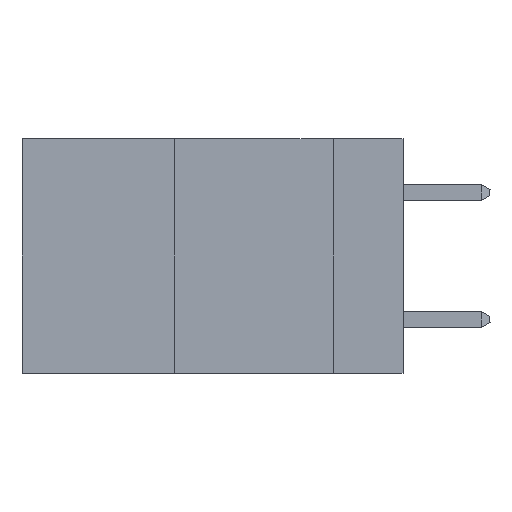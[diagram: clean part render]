
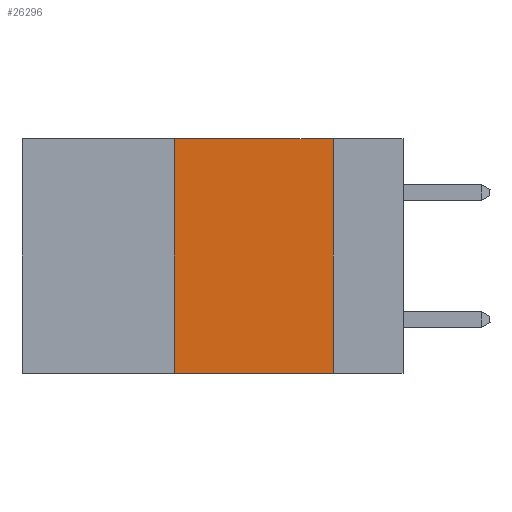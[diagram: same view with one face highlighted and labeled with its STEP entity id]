
A CAD part, left-side view. The second image highlights one B-rep face of the part: STEP entity #26296.
In plain terms, the highlighted planar face has unit normal (-1, 0, 0).
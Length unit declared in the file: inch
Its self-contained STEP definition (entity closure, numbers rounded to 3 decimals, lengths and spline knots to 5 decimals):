
#420 = LINE ( 'NONE', #38541, #2342 ) ;
#557 = FACE_OUTER_BOUND ( 'NONE', #25082, .T. ) ;
#2268 = CARTESIAN_POINT ( 'NONE',  ( 0., 0.11, 0. ) ) ;
#2342 = VECTOR ( 'NONE', #4422, 39.37008 ) ;
#3416 = DIRECTION ( 'NONE',  ( 0., -1., 0. ) ) ;
#4422 = DIRECTION ( 'NONE',  ( 0., 0., 1. ) ) ;
#5061 = DIRECTION ( 'NONE',  ( 0., 0., -1. ) ) ;
#5776 = VERTEX_POINT ( 'NONE', #28253 ) ;
#6001 = VERTEX_POINT ( 'NONE', #20505 ) ;
#7867 = EDGE_CURVE ( 'NONE', #28343, #23817, #420, .T. ) ;
#9557 = CARTESIAN_POINT ( 'NONE',  ( 0., 0.6, 0. ) ) ;
#10523 = ORIENTED_EDGE ( 'NONE', *, *, #34830, .F. ) ;
#14148 = ORIENTED_EDGE ( 'NONE', *, *, #7867, .F. ) ;
#15037 = VECTOR ( 'NONE', #29779, 39.37008 ) ;
#17250 = PLANE ( 'NONE',  #29747 ) ;
#18800 = ORIENTED_EDGE ( 'NONE', *, *, #27921, .T. ) ;
#20505 = CARTESIAN_POINT ( 'NONE',  ( 0., 0.11, 0. ) ) ;
#21212 = EDGE_CURVE ( 'NONE', #6001, #5776, #23116, .T. ) ;
#23116 = LINE ( 'NONE', #2268, #15037 ) ;
#23328 = DIRECTION ( 'NONE',  ( 1., 0., 0. ) ) ;
#23702 = CARTESIAN_POINT ( 'NONE',  ( 0., 0.6, -0.37 ) ) ;
#23817 = VERTEX_POINT ( 'NONE', #29712 ) ;
#25082 = EDGE_LOOP ( 'NONE', ( #25515, #10523, #14148, #18800 ) ) ;
#25515 = ORIENTED_EDGE ( 'NONE', *, *, #21212, .F. ) ;
#26296 = ADVANCED_FACE ( 'NONE', ( #557 ), #17250, .F. ) ;
#27921 = EDGE_CURVE ( 'NONE', #28343, #5776, #33883, .T. ) ;
#28253 = CARTESIAN_POINT ( 'NONE',  ( 0., 0.11, -0.37 ) ) ;
#28343 = VERTEX_POINT ( 'NONE', #34662 ) ;
#29712 = CARTESIAN_POINT ( 'NONE',  ( 0., 0.36, 0. ) ) ;
#29747 = AXIS2_PLACEMENT_3D ( 'NONE', #29761, #23328, #5061 ) ;
#29761 = CARTESIAN_POINT ( 'NONE',  ( 0., 0.6, 0. ) ) ;
#29779 = DIRECTION ( 'NONE',  ( 0., 0., -1. ) ) ;
#29919 = VECTOR ( 'NONE', #3416, 39.37008 ) ;
#30055 = VECTOR ( 'NONE', #35729, 39.37008 ) ;
#33883 = LINE ( 'NONE', #23702, #30055 ) ;
#34662 = CARTESIAN_POINT ( 'NONE',  ( 0., 0.36, -0.37 ) ) ;
#34830 = EDGE_CURVE ( 'NONE', #23817, #6001, #36085, .T. ) ;
#35729 = DIRECTION ( 'NONE',  ( 0., -1., 0. ) ) ;
#36085 = LINE ( 'NONE', #9557, #29919 ) ;
#38541 = CARTESIAN_POINT ( 'NONE',  ( 0., 0.36, 0. ) ) ;
